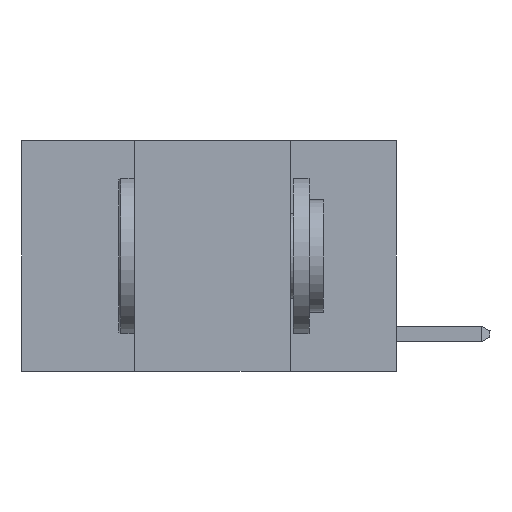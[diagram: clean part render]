
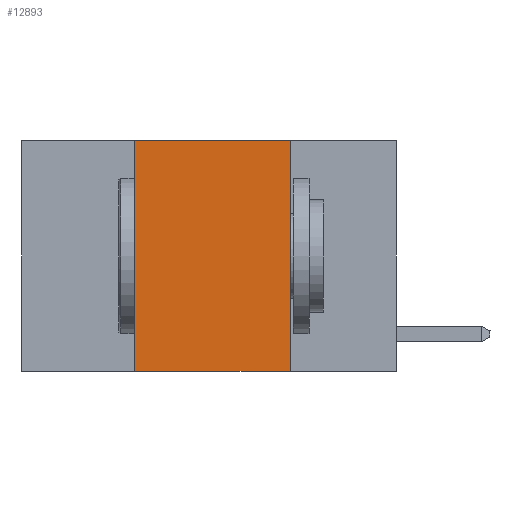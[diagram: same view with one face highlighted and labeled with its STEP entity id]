
A CAD part, left-side view. The second image highlights one B-rep face of the part: STEP entity #12893.
In plain terms, the highlighted planar face has unit normal (-1, 0, 0).
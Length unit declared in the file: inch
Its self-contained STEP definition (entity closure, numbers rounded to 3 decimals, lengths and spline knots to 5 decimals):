
#285 = VECTOR ( 'NONE', #11492, 39.37008 ) ;
#434 = VERTEX_POINT ( 'NONE', #9617 ) ;
#862 = VERTEX_POINT ( 'NONE', #4245 ) ;
#1299 = VECTOR ( 'NONE', #13423, 39.37008 ) ;
#1355 = LINE ( 'NONE', #2442, #12792 ) ;
#1900 = VERTEX_POINT ( 'NONE', #9790 ) ;
#2442 = CARTESIAN_POINT ( 'NONE',  ( 0., 0.17, 0. ) ) ;
#3597 = ORIENTED_EDGE ( 'NONE', *, *, #10577, .F. ) ;
#4245 = CARTESIAN_POINT ( 'NONE',  ( 0., 0.17, -0.37 ) ) ;
#4583 = EDGE_CURVE ( 'NONE', #11642, #862, #17333, .T. ) ;
#5245 = FACE_OUTER_BOUND ( 'NONE', #13395, .T. ) ;
#5951 = ORIENTED_EDGE ( 'NONE', *, *, #14442, .F. ) ;
#6587 = PLANE ( 'NONE',  #8776 ) ;
#7519 = CARTESIAN_POINT ( 'NONE',  ( 0., 0.42, 0. ) ) ;
#7570 = CARTESIAN_POINT ( 'NONE',  ( 0., 0.6, 0. ) ) ;
#7580 = VECTOR ( 'NONE', #8953, 39.37008 ) ;
#8008 = CARTESIAN_POINT ( 'NONE',  ( 0., 0.6, -0.37 ) ) ;
#8776 = AXIS2_PLACEMENT_3D ( 'NONE', #10598, #15743, #12014 ) ;
#8862 = ORIENTED_EDGE ( 'NONE', *, *, #4583, .T. ) ;
#8941 = ORIENTED_EDGE ( 'NONE', *, *, #16548, .F. ) ;
#8953 = DIRECTION ( 'NONE',  ( 0., 0., 1. ) ) ;
#9617 = CARTESIAN_POINT ( 'NONE',  ( 0., 0.17, 0. ) ) ;
#9790 = CARTESIAN_POINT ( 'NONE',  ( 0., 0.42, 0. ) ) ;
#10412 = CARTESIAN_POINT ( 'NONE',  ( 0., 0.42, -0.37 ) ) ;
#10577 = EDGE_CURVE ( 'NONE', #11642, #1900, #11629, .T. ) ;
#10598 = CARTESIAN_POINT ( 'NONE',  ( 0., 0.6, 0. ) ) ;
#11492 = DIRECTION ( 'NONE',  ( 0., -1., 0. ) ) ;
#11587 = LINE ( 'NONE', #7570, #285 ) ;
#11629 = LINE ( 'NONE', #7519, #7580 ) ;
#11642 = VERTEX_POINT ( 'NONE', #10412 ) ;
#12014 = DIRECTION ( 'NONE',  ( 0., 0., -1. ) ) ;
#12792 = VECTOR ( 'NONE', #13555, 39.37008 ) ;
#12893 = ADVANCED_FACE ( 'NONE', ( #5245 ), #6587, .F. ) ;
#13395 = EDGE_LOOP ( 'NONE', ( #5951, #8941, #3597, #8862 ) ) ;
#13423 = DIRECTION ( 'NONE',  ( 0., -1., 0. ) ) ;
#13555 = DIRECTION ( 'NONE',  ( 0., 0., -1. ) ) ;
#14442 = EDGE_CURVE ( 'NONE', #434, #862, #1355, .T. ) ;
#15743 = DIRECTION ( 'NONE',  ( 1., 0., 0. ) ) ;
#16548 = EDGE_CURVE ( 'NONE', #1900, #434, #11587, .T. ) ;
#17333 = LINE ( 'NONE', #8008, #1299 ) ;
